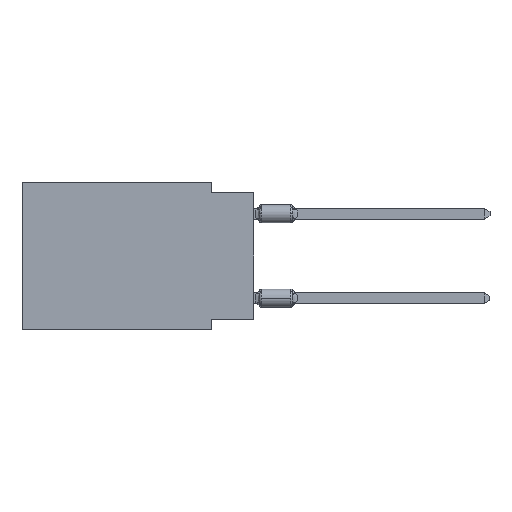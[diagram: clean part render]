
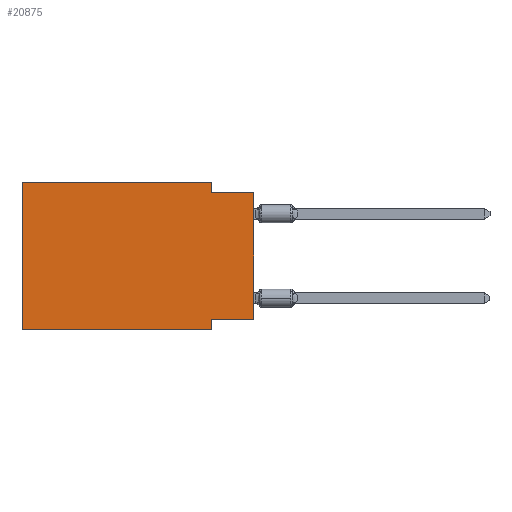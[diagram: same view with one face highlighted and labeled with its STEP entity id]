
A CAD part, left-side view. The second image highlights one B-rep face of the part: STEP entity #20875.
In plain terms, the highlighted planar face has unit normal (-1, 0, 0).
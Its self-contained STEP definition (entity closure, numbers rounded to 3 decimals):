
#330 = FACE_OUTER_BOUND ( 'NONE', #13701, .T. ) ;
#887 = LINE ( 'NONE', #4093, #8574 ) ;
#1331 = DIRECTION ( 'NONE',  ( 0., -1., 0. ) ) ;
#1333 = CARTESIAN_POINT ( 'NONE',  ( 0., 2.54, -8.89 ) ) ;
#2592 = VECTOR ( 'NONE', #16223, 1000. ) ;
#2788 = VERTEX_POINT ( 'NONE', #1333 ) ;
#3137 = LINE ( 'NONE', #16131, #7430 ) ;
#3311 = DIRECTION ( 'NONE',  ( 0., 0., 1. ) ) ;
#3421 = LINE ( 'NONE', #10884, #6422 ) ;
#3751 = LINE ( 'NONE', #13068, #16962 ) ;
#4093 = CARTESIAN_POINT ( 'NONE',  ( 0., 0., -0.635 ) ) ;
#4380 = CARTESIAN_POINT ( 'NONE',  ( 0., 13.97, 0. ) ) ;
#4432 = LINE ( 'NONE', #18277, #15168 ) ;
#4457 = DIRECTION ( 'NONE',  ( 0., -1., 0. ) ) ;
#4738 = VERTEX_POINT ( 'NONE', #16803 ) ;
#5406 = EDGE_CURVE ( 'NONE', #20783, #4738, #3137, .T. ) ;
#5788 = EDGE_CURVE ( 'NONE', #15576, #2788, #15502, .T. ) ;
#5848 = ORIENTED_EDGE ( 'NONE', *, *, #24011, .F. ) ;
#5966 = ORIENTED_EDGE ( 'NONE', *, *, #10502, .F. ) ;
#6302 = DIRECTION ( 'NONE',  ( 0., 0., -1. ) ) ;
#6422 = VECTOR ( 'NONE', #1331, 1000. ) ;
#7080 = CARTESIAN_POINT ( 'NONE',  ( 0., 13.97, -8.89 ) ) ;
#7208 = ORIENTED_EDGE ( 'NONE', *, *, #5406, .F. ) ;
#7430 = VECTOR ( 'NONE', #21794, 1000. ) ;
#7754 = ORIENTED_EDGE ( 'NONE', *, *, #20936, .F. ) ;
#8046 = DIRECTION ( 'NONE',  ( 1., 0., 0. ) ) ;
#8298 = VERTEX_POINT ( 'NONE', #10555 ) ;
#8574 = VECTOR ( 'NONE', #4457, 1000. ) ;
#8736 = CARTESIAN_POINT ( 'NONE',  ( 0., 0., -8.255 ) ) ;
#9610 = CARTESIAN_POINT ( 'NONE',  ( 0., 2.54, -8.89 ) ) ;
#9939 = AXIS2_PLACEMENT_3D ( 'NONE', #4380, #8046, #21068 ) ;
#9994 = EDGE_CURVE ( 'NONE', #20783, #2788, #3421, .T. ) ;
#10502 = EDGE_CURVE ( 'NONE', #4738, #18650, #3751, .T. ) ;
#10555 = CARTESIAN_POINT ( 'NONE',  ( 0., 0., -0.635 ) ) ;
#10607 = LINE ( 'NONE', #16135, #17414 ) ;
#10884 = CARTESIAN_POINT ( 'NONE',  ( 0., 13.97, -8.89 ) ) ;
#11174 = LINE ( 'NONE', #8736, #2592 ) ;
#11372 = VECTOR ( 'NONE', #6302, 1000. ) ;
#13068 = CARTESIAN_POINT ( 'NONE',  ( 0., 13.97, 0. ) ) ;
#13701 = EDGE_LOOP ( 'NONE', ( #23043, #5848, #7754, #5966, #7208, #17682, #16250, #19405 ) ) ;
#14549 = EDGE_CURVE ( 'NONE', #17281, #8298, #4432, .T. ) ;
#15104 = CARTESIAN_POINT ( 'NONE',  ( 0., 0., -8.255 ) ) ;
#15168 = VECTOR ( 'NONE', #3311, 1000. ) ;
#15502 = LINE ( 'NONE', #9610, #11372 ) ;
#15576 = VERTEX_POINT ( 'NONE', #16242 ) ;
#16131 = CARTESIAN_POINT ( 'NONE',  ( 0., 13.97, 0. ) ) ;
#16135 = CARTESIAN_POINT ( 'NONE',  ( 0., 2.54, 0. ) ) ;
#16223 = DIRECTION ( 'NONE',  ( 0., 1., 0. ) ) ;
#16242 = CARTESIAN_POINT ( 'NONE',  ( 0., 2.54, -8.255 ) ) ;
#16250 = ORIENTED_EDGE ( 'NONE', *, *, #5788, .F. ) ;
#16803 = CARTESIAN_POINT ( 'NONE',  ( 0., 13.97, 0. ) ) ;
#16962 = VECTOR ( 'NONE', #18362, 1000. ) ;
#17281 = VERTEX_POINT ( 'NONE', #15104 ) ;
#17414 = VECTOR ( 'NONE', #21566, 1000. ) ;
#17500 = PLANE ( 'NONE',  #9939 ) ;
#17682 = ORIENTED_EDGE ( 'NONE', *, *, #9994, .T. ) ;
#18277 = CARTESIAN_POINT ( 'NONE',  ( 0., 0., 0. ) ) ;
#18362 = DIRECTION ( 'NONE',  ( 0., -1., 0. ) ) ;
#18452 = EDGE_CURVE ( 'NONE', #17281, #15576, #11174, .T. ) ;
#18565 = CARTESIAN_POINT ( 'NONE',  ( 0., 2.54, -0.635 ) ) ;
#18650 = VERTEX_POINT ( 'NONE', #21373 ) ;
#19405 = ORIENTED_EDGE ( 'NONE', *, *, #18452, .F. ) ;
#20783 = VERTEX_POINT ( 'NONE', #7080 ) ;
#20875 = ADVANCED_FACE ( 'NONE', ( #330 ), #17500, .F. ) ;
#20936 = EDGE_CURVE ( 'NONE', #18650, #22680, #10607, .T. ) ;
#21068 = DIRECTION ( 'NONE',  ( 0., 0., -1. ) ) ;
#21373 = CARTESIAN_POINT ( 'NONE',  ( 0., 2.54, 0. ) ) ;
#21566 = DIRECTION ( 'NONE',  ( 0., 0., -1. ) ) ;
#21794 = DIRECTION ( 'NONE',  ( 0., 0., 1. ) ) ;
#22680 = VERTEX_POINT ( 'NONE', #18565 ) ;
#23043 = ORIENTED_EDGE ( 'NONE', *, *, #14549, .T. ) ;
#24011 = EDGE_CURVE ( 'NONE', #22680, #8298, #887, .T. ) ;
